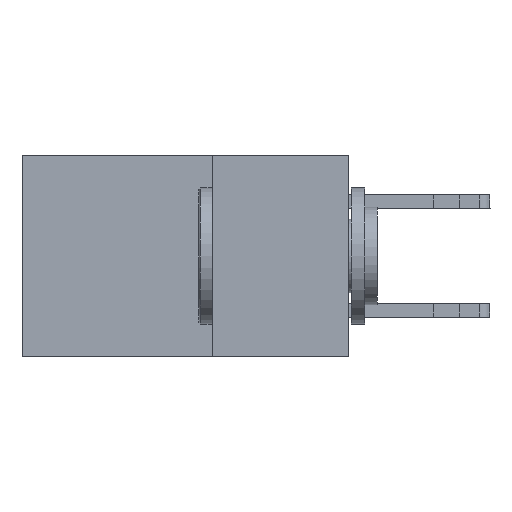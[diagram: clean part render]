
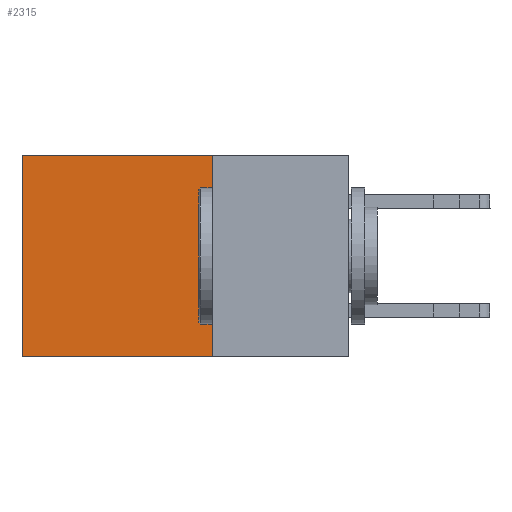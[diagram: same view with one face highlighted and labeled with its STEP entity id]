
A CAD part, left-side view. The second image highlights one B-rep face of the part: STEP entity #2315.
In plain terms, the highlighted planar face has unit normal (-1, 0, 0).
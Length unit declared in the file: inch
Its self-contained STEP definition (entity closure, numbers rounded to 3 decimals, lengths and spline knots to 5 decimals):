
#46 = DIRECTION ( 'NONE',  ( 0., 0., -1. ) ) ;
#170 = CARTESIAN_POINT ( 'NONE',  ( 0.2615, 0.25, -0.37 ) ) ;
#541 = ORIENTED_EDGE ( 'NONE', *, *, #1009, .T. ) ;
#692 = DIRECTION ( 'NONE',  ( 0., 1., 0. ) ) ;
#1009 = EDGE_CURVE ( 'NONE', #8175, #9344, #5617, .T. ) ;
#1113 = DIRECTION ( 'NONE',  ( 0., 0., -1. ) ) ;
#1526 = EDGE_CURVE ( 'NONE', #6272, #10322, #10426, .T. ) ;
#1712 = EDGE_CURVE ( 'NONE', #9344, #10322, #10598, .T. ) ;
#2315 = ADVANCED_FACE ( 'NONE', ( #7694 ), #7806, .F. ) ;
#2744 = CARTESIAN_POINT ( 'NONE',  ( 0.2615, 0.25, -0.37 ) ) ;
#3913 = EDGE_CURVE ( 'NONE', #8175, #6272, #7356, .T. ) ;
#4216 = CARTESIAN_POINT ( 'NONE',  ( 0.2615, 0.25, -0.37 ) ) ;
#4475 = VECTOR ( 'NONE', #5301, 39.37008 ) ;
#4560 = ORIENTED_EDGE ( 'NONE', *, *, #1712, .T. ) ;
#4907 = VECTOR ( 'NONE', #1113, 39.37008 ) ;
#5261 = ORIENTED_EDGE ( 'NONE', *, *, #3913, .F. ) ;
#5301 = DIRECTION ( 'NONE',  ( 0., 0., -1. ) ) ;
#5413 = CARTESIAN_POINT ( 'NONE',  ( 0.2615, 0.6, -0.37 ) ) ;
#5617 = LINE ( 'NONE', #9143, #10874 ) ;
#6272 = VERTEX_POINT ( 'NONE', #170 ) ;
#6899 = DIRECTION ( 'NONE',  ( 1., 0., 0. ) ) ;
#7135 = EDGE_LOOP ( 'NONE', ( #4560, #8046, #5261, #541 ) ) ;
#7356 = LINE ( 'NONE', #8874, #4907 ) ;
#7425 = DIRECTION ( 'NONE',  ( 0., 1., 0. ) ) ;
#7463 = CARTESIAN_POINT ( 'NONE',  ( 0.2615, 0.25, 0. ) ) ;
#7694 = FACE_OUTER_BOUND ( 'NONE', #7135, .T. ) ;
#7806 = PLANE ( 'NONE',  #7888 ) ;
#7883 = VECTOR ( 'NONE', #692, 39.37008 ) ;
#7888 = AXIS2_PLACEMENT_3D ( 'NONE', #2744, #6899, #46 ) ;
#8046 = ORIENTED_EDGE ( 'NONE', *, *, #1526, .F. ) ;
#8175 = VERTEX_POINT ( 'NONE', #7463 ) ;
#8874 = CARTESIAN_POINT ( 'NONE',  ( 0.2615, 0.25, -0.37 ) ) ;
#8908 = CARTESIAN_POINT ( 'NONE',  ( 0.2615, 0.6, -0.37 ) ) ;
#9143 = CARTESIAN_POINT ( 'NONE',  ( 0.2615, 0.25, 0. ) ) ;
#9344 = VERTEX_POINT ( 'NONE', #10674 ) ;
#10322 = VERTEX_POINT ( 'NONE', #5413 ) ;
#10426 = LINE ( 'NONE', #4216, #7883 ) ;
#10598 = LINE ( 'NONE', #8908, #4475 ) ;
#10674 = CARTESIAN_POINT ( 'NONE',  ( 0.2615, 0.6, 0. ) ) ;
#10874 = VECTOR ( 'NONE', #7425, 39.37008 ) ;
